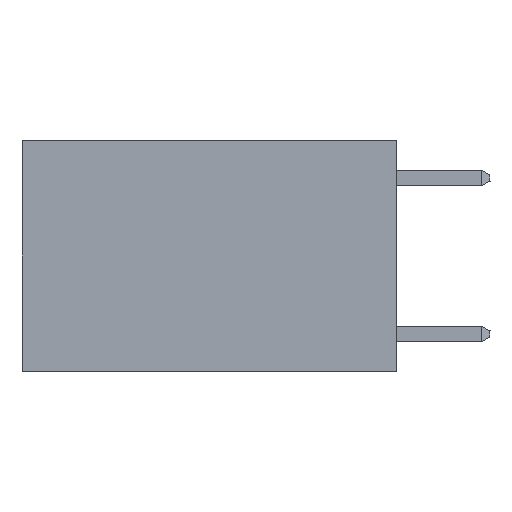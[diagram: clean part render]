
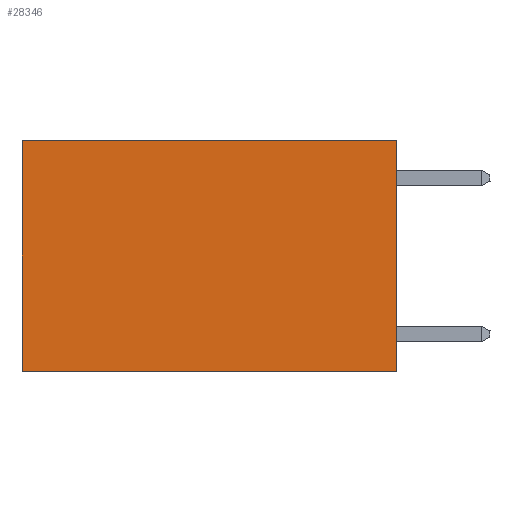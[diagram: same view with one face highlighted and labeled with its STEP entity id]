
A CAD part, left-side view. The second image highlights one B-rep face of the part: STEP entity #28346.
In plain terms, the highlighted planar face has unit normal (-1, 0, 0).
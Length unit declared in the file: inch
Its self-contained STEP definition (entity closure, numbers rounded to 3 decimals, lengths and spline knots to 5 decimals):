
#740 = ORIENTED_EDGE ( 'NONE', *, *, #24839, .F. ) ;
#968 = EDGE_LOOP ( 'NONE', ( #14521, #740, #21209, #28677 ) ) ;
#1052 = CARTESIAN_POINT ( 'NONE',  ( 0.2625, 0., 0. ) ) ;
#1269 = FACE_OUTER_BOUND ( 'NONE', #968, .T. ) ;
#2129 = VECTOR ( 'NONE', #10089, 39.37008 ) ;
#3332 = PLANE ( 'NONE',  #7104 ) ;
#3611 = VERTEX_POINT ( 'NONE', #19862 ) ;
#7104 = AXIS2_PLACEMENT_3D ( 'NONE', #16525, #21005, #12515 ) ;
#7955 = LINE ( 'NONE', #16976, #17345 ) ;
#8361 = LINE ( 'NONE', #24359, #23083 ) ;
#9282 = CARTESIAN_POINT ( 'NONE',  ( 0.2625, 0., 0. ) ) ;
#10013 = EDGE_CURVE ( 'NONE', #28233, #17648, #12290, .T. ) ;
#10089 = DIRECTION ( 'NONE',  ( 0., 0., -1. ) ) ;
#11796 = DIRECTION ( 'NONE',  ( 0., 1., 0. ) ) ;
#12290 = LINE ( 'NONE', #1052, #2129 ) ;
#12301 = VECTOR ( 'NONE', #22860, 39.37008 ) ;
#12515 = DIRECTION ( 'NONE',  ( 0., 0., -1. ) ) ;
#14521 = ORIENTED_EDGE ( 'NONE', *, *, #28722, .T. ) ;
#16525 = CARTESIAN_POINT ( 'NONE',  ( 0.2625, 0., 0. ) ) ;
#16976 = CARTESIAN_POINT ( 'NONE',  ( 0.2625, 0., 0. ) ) ;
#17345 = VECTOR ( 'NONE', #11796, 39.37008 ) ;
#17648 = VERTEX_POINT ( 'NONE', #18596 ) ;
#18596 = CARTESIAN_POINT ( 'NONE',  ( 0.2625, 0., -0.37 ) ) ;
#18851 = CARTESIAN_POINT ( 'NONE',  ( 0.2625, 0.6, 0. ) ) ;
#19862 = CARTESIAN_POINT ( 'NONE',  ( 0.2625, 0.6, 0. ) ) ;
#20893 = CARTESIAN_POINT ( 'NONE',  ( 0.2625, 0.6, -0.37 ) ) ;
#21005 = DIRECTION ( 'NONE',  ( 1., 0., 0. ) ) ;
#21209 = ORIENTED_EDGE ( 'NONE', *, *, #10013, .F. ) ;
#21845 = DIRECTION ( 'NONE',  ( 0., 1., 0. ) ) ;
#22860 = DIRECTION ( 'NONE',  ( 0., 0., -1. ) ) ;
#23083 = VECTOR ( 'NONE', #21845, 39.37008 ) ;
#24286 = EDGE_CURVE ( 'NONE', #28233, #3611, #7955, .T. ) ;
#24359 = CARTESIAN_POINT ( 'NONE',  ( 0.2625, 0., -0.37 ) ) ;
#24839 = EDGE_CURVE ( 'NONE', #17648, #27765, #8361, .T. ) ;
#27433 = LINE ( 'NONE', #18851, #12301 ) ;
#27765 = VERTEX_POINT ( 'NONE', #20893 ) ;
#28233 = VERTEX_POINT ( 'NONE', #9282 ) ;
#28346 = ADVANCED_FACE ( 'NONE', ( #1269 ), #3332, .F. ) ;
#28677 = ORIENTED_EDGE ( 'NONE', *, *, #24286, .T. ) ;
#28722 = EDGE_CURVE ( 'NONE', #3611, #27765, #27433, .T. ) ;
